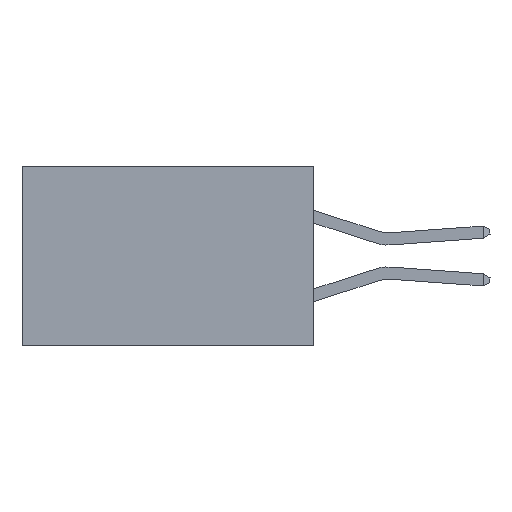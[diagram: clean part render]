
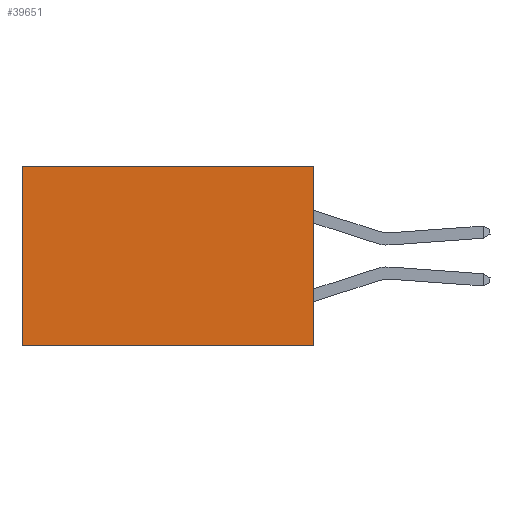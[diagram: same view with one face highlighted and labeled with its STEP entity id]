
A CAD part, left-side view. The second image highlights one B-rep face of the part: STEP entity #39651.
In plain terms, the highlighted planar face has unit normal (-1, 0, 0).
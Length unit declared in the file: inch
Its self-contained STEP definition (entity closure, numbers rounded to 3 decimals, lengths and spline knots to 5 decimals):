
#61 = VERTEX_POINT ( 'NONE', #2774 ) ;
#1851 = CARTESIAN_POINT ( 'NONE',  ( 0.2875, 0.6, 0. ) ) ;
#2774 = CARTESIAN_POINT ( 'NONE',  ( 0.2875, 0.6, 0. ) ) ;
#3854 = DIRECTION ( 'NONE',  ( 0., 0., -1. ) ) ;
#3959 = LINE ( 'NONE', #12633, #16272 ) ;
#4763 = CARTESIAN_POINT ( 'NONE',  ( 0.2875, 0., -0.37 ) ) ;
#5478 = ORIENTED_EDGE ( 'NONE', *, *, #8040, .T. ) ;
#6195 = ORIENTED_EDGE ( 'NONE', *, *, #22021, .F. ) ;
#6782 = EDGE_LOOP ( 'NONE', ( #31585, #14796, #6195, #5478 ) ) ;
#8040 = EDGE_CURVE ( 'NONE', #13950, #61, #40190, .T. ) ;
#8061 = PLANE ( 'NONE',  #22482 ) ;
#8600 = VECTOR ( 'NONE', #11728, 39.37008 ) ;
#9631 = FACE_OUTER_BOUND ( 'NONE', #6782, .T. ) ;
#11506 = CARTESIAN_POINT ( 'NONE',  ( 0.2875, 0., 0. ) ) ;
#11635 = DIRECTION ( 'NONE',  ( 0., 0., -1. ) ) ;
#11728 = DIRECTION ( 'NONE',  ( 0., 0., -1. ) ) ;
#12633 = CARTESIAN_POINT ( 'NONE',  ( 0.2875, 0., 0. ) ) ;
#13950 = VERTEX_POINT ( 'NONE', #18934 ) ;
#14796 = ORIENTED_EDGE ( 'NONE', *, *, #39049, .F. ) ;
#16272 = VECTOR ( 'NONE', #3854, 39.37008 ) ;
#16605 = LINE ( 'NONE', #33927, #31832 ) ;
#18934 = CARTESIAN_POINT ( 'NONE',  ( 0.2875, 0., 0. ) ) ;
#19710 = VERTEX_POINT ( 'NONE', #4763 ) ;
#20537 = DIRECTION ( 'NONE',  ( 0., 1., 0. ) ) ;
#22021 = EDGE_CURVE ( 'NONE', #13950, #19710, #3959, .T. ) ;
#22482 = AXIS2_PLACEMENT_3D ( 'NONE', #11506, #39466, #11635 ) ;
#23245 = VERTEX_POINT ( 'NONE', #37926 ) ;
#26736 = CARTESIAN_POINT ( 'NONE',  ( 0.2875, 0., 0. ) ) ;
#28786 = LINE ( 'NONE', #1851, #8600 ) ;
#31585 = ORIENTED_EDGE ( 'NONE', *, *, #40385, .T. ) ;
#31832 = VECTOR ( 'NONE', #37198, 39.37008 ) ;
#33927 = CARTESIAN_POINT ( 'NONE',  ( 0.2875, 0., -0.37 ) ) ;
#35382 = VECTOR ( 'NONE', #20537, 39.37008 ) ;
#37198 = DIRECTION ( 'NONE',  ( 0., 1., 0. ) ) ;
#37926 = CARTESIAN_POINT ( 'NONE',  ( 0.2875, 0.6, -0.37 ) ) ;
#39049 = EDGE_CURVE ( 'NONE', #19710, #23245, #16605, .T. ) ;
#39466 = DIRECTION ( 'NONE',  ( 1., 0., 0. ) ) ;
#39651 = ADVANCED_FACE ( 'NONE', ( #9631 ), #8061, .F. ) ;
#40190 = LINE ( 'NONE', #26736, #35382 ) ;
#40385 = EDGE_CURVE ( 'NONE', #61, #23245, #28786, .T. ) ;
